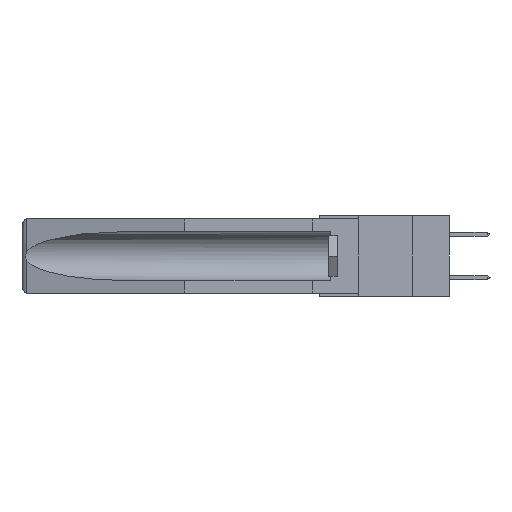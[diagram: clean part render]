
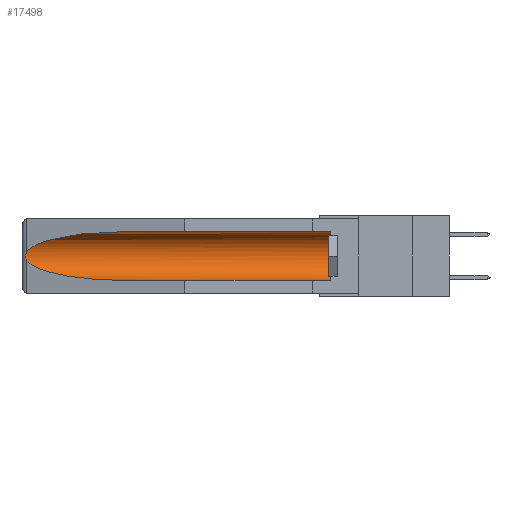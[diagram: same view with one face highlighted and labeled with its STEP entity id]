
A CAD part, left-side view. The second image highlights one B-rep face of the part: STEP entity #17498.
In plain terms, the highlighted cylindrical face has radius 2.857 mm (diameter 5.715 mm), a partial arc.
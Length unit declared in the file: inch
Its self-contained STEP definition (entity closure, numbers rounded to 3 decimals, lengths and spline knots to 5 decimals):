
#245 = ORIENTED_EDGE ( 'NONE', *, *, #22354, .T. ) ;
#575 = DIRECTION ( 'NONE',  ( 0., 0., 1. ) ) ;
#613 = CARTESIAN_POINT ( 'NONE',  ( 0.2675, 1.53308, -0.16763 ) ) ;
#661 = ORIENTED_EDGE ( 'NONE', *, *, #1731, .T. ) ;
#1487 = ORIENTED_EDGE ( 'NONE', *, *, #6731, .T. ) ;
#1731 = EDGE_CURVE ( 'NONE', #25485, #2325, #16449, .T. ) ;
#1833 = CARTESIAN_POINT ( 'NONE',  ( 0.155, 1.07973, -0.284 ) ) ;
#1992 = VECTOR ( 'NONE', #3635, 39.37008 ) ;
#2325 = VERTEX_POINT ( 'NONE', #9068 ) ;
#2677 = CARTESIAN_POINT ( 'NONE',  ( 0.21114, 1.30732, -0.059 ) ) ;
#2740 = DIRECTION ( 'NONE',  ( 0., 1., 0. ) ) ;
#3081 = CARTESIAN_POINT ( 'NONE',  ( 0.26655, 1.53094, -0.18657 ) ) ;
#3365 = EDGE_CURVE ( 'NONE', #11520, #22564, #27039, .T. ) ;
#3635 = DIRECTION ( 'NONE',  ( 0., 1., 0. ) ) ;
#3637 = CARTESIAN_POINT ( 'NONE',  ( 0.21114, 1.30732, -0.284 ) ) ;
#3842 = LINE ( 'NONE', #16352, #13082 ) ;
#4999 =( BOUNDED_CURVE ( )  B_SPLINE_CURVE ( 3, ( #27533, #2677, #18670, #17858 ),
 .UNSPECIFIED., .F., .F. ) 
 B_SPLINE_CURVE_WITH_KNOTS ( ( 4, 4 ),
 ( 4.71239, 6.08839 ),
 .UNSPECIFIED. ) 
 CURVE ( )  GEOMETRIC_REPRESENTATION_ITEM ( )  RATIONAL_B_SPLINE_CURVE ( ( 1., 0.848, 0.848, 1. ) ) 
 REPRESENTATION_ITEM ( '' )  );
#6091 = VERTEX_POINT ( 'NONE', #6838 ) ;
#6731 = EDGE_CURVE ( 'NONE', #6091, #25485, #4999, .T. ) ;
#6838 = CARTESIAN_POINT ( 'NONE',  ( 0.155, 1.07973, -0.059 ) ) ;
#9068 = CARTESIAN_POINT ( 'NONE',  ( 0.26537, 1.52718, -0.19328 ) ) ;
#10125 = CYLINDRICAL_SURFACE ( 'NONE', #10942, 0.1125 ) ;
#10833 = FACE_OUTER_BOUND ( 'NONE', #25027, .T. ) ;
#10942 = AXIS2_PLACEMENT_3D ( 'NONE', #11559, #16425, #18709 ) ;
#11520 = VERTEX_POINT ( 'NONE', #15615 ) ;
#11559 = CARTESIAN_POINT ( 'NONE',  ( 0.155, -0.30754, -0.1715 ) ) ;
#12019 = CARTESIAN_POINT ( 'NONE',  ( 0.155, 0.126, -0.1715 ) ) ;
#12056 = CARTESIAN_POINT ( 'NONE',  ( 0.2673, 1.5327, -0.16383 ) ) ;
#12220 = DIRECTION ( 'NONE',  ( 0., -1., 0. ) ) ;
#13082 = VECTOR ( 'NONE', #2740, 39.37008 ) ;
#13886 = ORIENTED_EDGE ( 'NONE', *, *, #3365, .T. ) ;
#14079 = LINE ( 'NONE', #21943, #1992 ) ;
#14102 = CARTESIAN_POINT ( 'NONE',  ( 0.26537, 1.52718, -0.19328 ) ) ;
#14421 = CARTESIAN_POINT ( 'NONE',  ( 0.2675, 1.53308, -0.17534 ) ) ;
#15417 = CARTESIAN_POINT ( 'NONE',  ( 0.155, 0.126, -0.059 ) ) ;
#15615 = CARTESIAN_POINT ( 'NONE',  ( 0.155, 0.126, -0.284 ) ) ;
#16352 = CARTESIAN_POINT ( 'NONE',  ( 0.155, -0.30754, -0.059 ) ) ;
#16425 = DIRECTION ( 'NONE',  ( 0., 1., 0. ) ) ;
#16449 = B_SPLINE_CURVE_WITH_KNOTS ( 'NONE', 3,
 ( #23483, #25756, #18781, #12056, #613, #14421, #16491, #3081, #25464, #18976 ),
 .UNSPECIFIED., .F., .F.,
 ( 4, 2, 2, 2, 4 ),
 ( 0., 0.00029, 0.00058, 0.00087, 0.00117 ),
 .UNSPECIFIED. ) ;
#16491 = CARTESIAN_POINT ( 'NONE',  ( 0.2673, 1.53269, -0.17917 ) ) ;
#17361 = AXIS2_PLACEMENT_3D ( 'NONE', #12019, #12220, #575 ) ;
#17498 = ADVANCED_FACE ( 'NONE', ( #10833 ), #10125, .F. ) ;
#17858 = CARTESIAN_POINT ( 'NONE',  ( 0.26537, 1.52718, -0.14972 ) ) ;
#18452 = CARTESIAN_POINT ( 'NONE',  ( 0.25451, 1.48313, -0.24835 ) ) ;
#18670 = CARTESIAN_POINT ( 'NONE',  ( 0.25451, 1.48313, -0.09465 ) ) ;
#18709 = DIRECTION ( 'NONE',  ( 0., 0., 1. ) ) ;
#18781 = CARTESIAN_POINT ( 'NONE',  ( 0.26654, 1.53092, -0.15636 ) ) ;
#18976 = CARTESIAN_POINT ( 'NONE',  ( 0.26537, 1.52718, -0.19328 ) ) ;
#19936 =( BOUNDED_CURVE ( )  B_SPLINE_CURVE ( 3, ( #14102, #18452, #3637, #1833 ),
 .UNSPECIFIED., .F., .F. ) 
 B_SPLINE_CURVE_WITH_KNOTS ( ( 4, 4 ),
 ( 0.1948, 1.5708 ),
 .UNSPECIFIED. ) 
 CURVE ( )  GEOMETRIC_REPRESENTATION_ITEM ( )  RATIONAL_B_SPLINE_CURVE ( ( 1., 0.848, 0.848, 1. ) ) 
 REPRESENTATION_ITEM ( '' )  );
#20103 = CARTESIAN_POINT ( 'NONE',  ( 0.155, 1.07973, -0.284 ) ) ;
#21943 = CARTESIAN_POINT ( 'NONE',  ( 0.155, -0.30754, -0.284 ) ) ;
#22354 = EDGE_CURVE ( 'NONE', #22564, #6091, #3842, .T. ) ;
#22564 = VERTEX_POINT ( 'NONE', #15417 ) ;
#22816 = ORIENTED_EDGE ( 'NONE', *, *, #28234, .T. ) ;
#23483 = CARTESIAN_POINT ( 'NONE',  ( 0.26537, 1.52718, -0.14972 ) ) ;
#25027 = EDGE_LOOP ( 'NONE', ( #1487, #661, #22816, #26516, #13886, #245 ) ) ;
#25052 = EDGE_CURVE ( 'NONE', #11520, #25229, #14079, .T. ) ;
#25229 = VERTEX_POINT ( 'NONE', #20103 ) ;
#25464 = CARTESIAN_POINT ( 'NONE',  ( 0.26597, 1.5296, -0.19026 ) ) ;
#25485 = VERTEX_POINT ( 'NONE', #25666 ) ;
#25666 = CARTESIAN_POINT ( 'NONE',  ( 0.26537, 1.52718, -0.14972 ) ) ;
#25756 = CARTESIAN_POINT ( 'NONE',  ( 0.26597, 1.52961, -0.15275 ) ) ;
#26516 = ORIENTED_EDGE ( 'NONE', *, *, #25052, .F. ) ;
#27039 = CIRCLE ( 'NONE', #17361, 0.1125 ) ;
#27533 = CARTESIAN_POINT ( 'NONE',  ( 0.155, 1.07973, -0.059 ) ) ;
#28234 = EDGE_CURVE ( 'NONE', #2325, #25229, #19936, .T. ) ;
